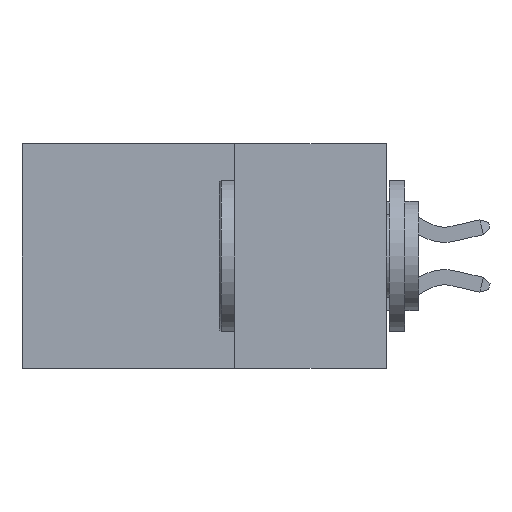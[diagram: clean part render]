
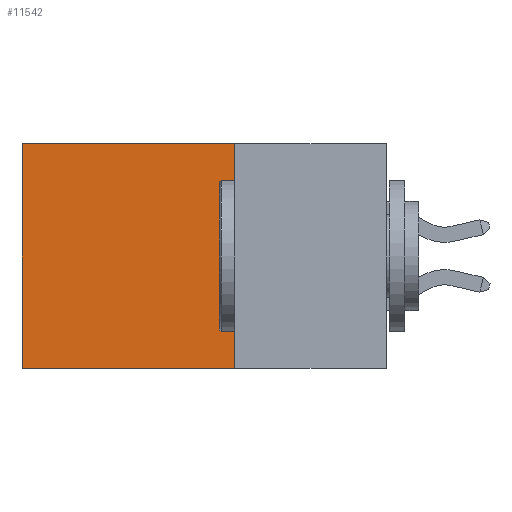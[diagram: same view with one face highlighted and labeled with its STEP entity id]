
A CAD part, left-side view. The second image highlights one B-rep face of the part: STEP entity #11542.
In plain terms, the highlighted planar face has unit normal (-1, 0, 0).
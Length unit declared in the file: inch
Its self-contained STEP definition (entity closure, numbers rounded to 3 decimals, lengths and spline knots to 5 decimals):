
#313 = DIRECTION ( 'NONE',  ( 0., 0., -1. ) ) ;
#324 = LINE ( 'NONE', #10387, #9688 ) ;
#990 = CARTESIAN_POINT ( 'NONE',  ( 0.2615, 0.25, -0.37 ) ) ;
#994 = DIRECTION ( 'NONE',  ( 1., 0., 0. ) ) ;
#1171 = PLANE ( 'NONE',  #6892 ) ;
#1258 = ORIENTED_EDGE ( 'NONE', *, *, #2997, .F. ) ;
#1619 = EDGE_CURVE ( 'NONE', #7841, #3230, #8439, .T. ) ;
#1752 = ORIENTED_EDGE ( 'NONE', *, *, #1806, .F. ) ;
#1806 = EDGE_CURVE ( 'NONE', #13497, #3230, #3085, .T. ) ;
#2488 = LINE ( 'NONE', #6489, #14070 ) ;
#2858 = DIRECTION ( 'NONE',  ( 0., 1., 0. ) ) ;
#2997 = EDGE_CURVE ( 'NONE', #3012, #13497, #2488, .T. ) ;
#3012 = VERTEX_POINT ( 'NONE', #5016 ) ;
#3085 = LINE ( 'NONE', #8517, #11523 ) ;
#3230 = VERTEX_POINT ( 'NONE', #9813 ) ;
#4567 = FACE_OUTER_BOUND ( 'NONE', #12053, .T. ) ;
#5016 = CARTESIAN_POINT ( 'NONE',  ( 0.2615, 0.25, 0. ) ) ;
#5375 = DIRECTION ( 'NONE',  ( 0., 0., -1. ) ) ;
#5779 = CARTESIAN_POINT ( 'NONE',  ( 0.2615, 0.6, -0.37 ) ) ;
#5804 = DIRECTION ( 'NONE',  ( 0., 0., -1. ) ) ;
#6489 = CARTESIAN_POINT ( 'NONE',  ( 0.2615, 0.25, -0.37 ) ) ;
#6892 = AXIS2_PLACEMENT_3D ( 'NONE', #990, #994, #313 ) ;
#7027 = ORIENTED_EDGE ( 'NONE', *, *, #1619, .T. ) ;
#7041 = EDGE_CURVE ( 'NONE', #3012, #7841, #324, .T. ) ;
#7695 = CARTESIAN_POINT ( 'NONE',  ( 0.2615, 0.25, -0.37 ) ) ;
#7841 = VERTEX_POINT ( 'NONE', #13391 ) ;
#8049 = ORIENTED_EDGE ( 'NONE', *, *, #7041, .T. ) ;
#8439 = LINE ( 'NONE', #5779, #11035 ) ;
#8517 = CARTESIAN_POINT ( 'NONE',  ( 0.2615, 0.25, -0.37 ) ) ;
#9688 = VECTOR ( 'NONE', #10340, 39.37008 ) ;
#9813 = CARTESIAN_POINT ( 'NONE',  ( 0.2615, 0.6, -0.37 ) ) ;
#10340 = DIRECTION ( 'NONE',  ( 0., 1., 0. ) ) ;
#10387 = CARTESIAN_POINT ( 'NONE',  ( 0.2615, 0.25, 0. ) ) ;
#11035 = VECTOR ( 'NONE', #5375, 39.37008 ) ;
#11523 = VECTOR ( 'NONE', #2858, 39.37008 ) ;
#11542 = ADVANCED_FACE ( 'NONE', ( #4567 ), #1171, .F. ) ;
#12053 = EDGE_LOOP ( 'NONE', ( #7027, #1752, #1258, #8049 ) ) ;
#13391 = CARTESIAN_POINT ( 'NONE',  ( 0.2615, 0.6, 0. ) ) ;
#13497 = VERTEX_POINT ( 'NONE', #7695 ) ;
#14070 = VECTOR ( 'NONE', #5804, 39.37008 ) ;
